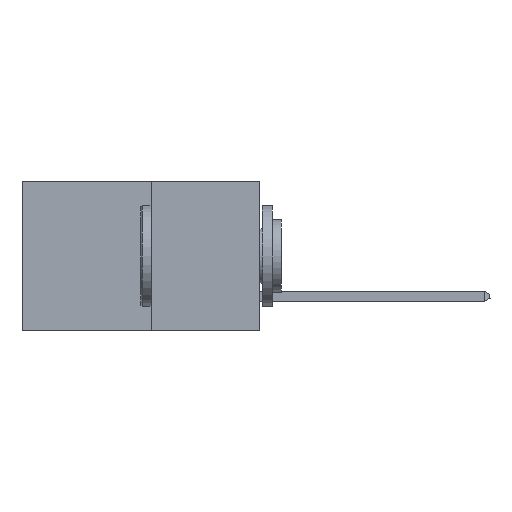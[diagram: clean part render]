
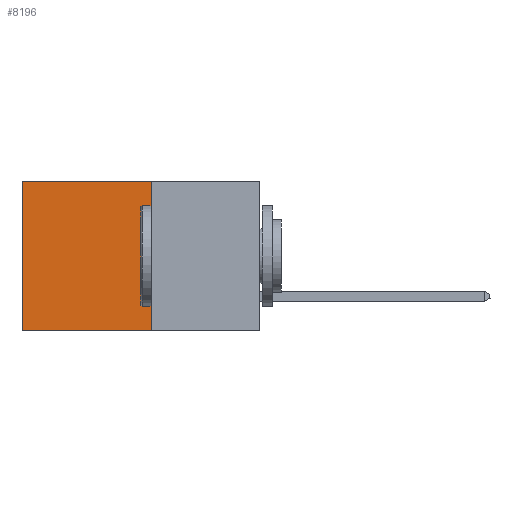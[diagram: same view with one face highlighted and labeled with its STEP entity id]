
A CAD part, left-side view. The second image highlights one B-rep face of the part: STEP entity #8196.
In plain terms, the highlighted planar face has unit normal (-1, 0, 0).
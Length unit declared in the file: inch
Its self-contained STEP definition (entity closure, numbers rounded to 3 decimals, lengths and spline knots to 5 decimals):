
#45 = CARTESIAN_POINT ( 'NONE',  ( 0.277, 0.27, 0. ) ) ;
#1614 = VECTOR ( 'NONE', #14670, 39.37008 ) ;
#1709 = CARTESIAN_POINT ( 'NONE',  ( 0.277, 0.59, 0. ) ) ;
#2320 = CARTESIAN_POINT ( 'NONE',  ( 0.277, 0.59, -0.37 ) ) ;
#2642 = EDGE_CURVE ( 'NONE', #5969, #11753, #12850, .T. ) ;
#2899 = EDGE_CURVE ( 'NONE', #5969, #7087, #11988, .T. ) ;
#3851 = EDGE_LOOP ( 'NONE', ( #8038, #6498, #10571, #11780 ) ) ;
#5511 = VERTEX_POINT ( 'NONE', #7799 ) ;
#5912 = DIRECTION ( 'NONE',  ( 0., 0., -1. ) ) ;
#5969 = VERTEX_POINT ( 'NONE', #14840 ) ;
#6498 = ORIENTED_EDGE ( 'NONE', *, *, #14004, .F. ) ;
#7087 = VERTEX_POINT ( 'NONE', #1709 ) ;
#7191 = FACE_OUTER_BOUND ( 'NONE', #3851, .T. ) ;
#7507 = CARTESIAN_POINT ( 'NONE',  ( 0.277, 0.27, -0.37 ) ) ;
#7799 = CARTESIAN_POINT ( 'NONE',  ( 0.277, 0.59, -0.37 ) ) ;
#8038 = ORIENTED_EDGE ( 'NONE', *, *, #17398, .T. ) ;
#8196 = ADVANCED_FACE ( 'NONE', ( #7191 ), #16973, .F. ) ;
#8259 = VECTOR ( 'NONE', #5912, 39.37008 ) ;
#10020 = AXIS2_PLACEMENT_3D ( 'NONE', #16842, #16813, #16790 ) ;
#10571 = ORIENTED_EDGE ( 'NONE', *, *, #2642, .F. ) ;
#11753 = VERTEX_POINT ( 'NONE', #13421 ) ;
#11780 = ORIENTED_EDGE ( 'NONE', *, *, #2899, .T. ) ;
#11988 = LINE ( 'NONE', #45, #16195 ) ;
#12850 = LINE ( 'NONE', #21275, #21290 ) ;
#13080 = LINE ( 'NONE', #2320, #8259 ) ;
#13421 = CARTESIAN_POINT ( 'NONE',  ( 0.277, 0.27, -0.37 ) ) ;
#14004 = EDGE_CURVE ( 'NONE', #11753, #5511, #16018, .T. ) ;
#14670 = DIRECTION ( 'NONE',  ( 0., 1., 0. ) ) ;
#14840 = CARTESIAN_POINT ( 'NONE',  ( 0.277, 0.27, 0. ) ) ;
#16018 = LINE ( 'NONE', #7507, #1614 ) ;
#16195 = VECTOR ( 'NONE', #19424, 39.37008 ) ;
#16790 = DIRECTION ( 'NONE',  ( 0., 0., -1. ) ) ;
#16813 = DIRECTION ( 'NONE',  ( 1., 0., 0. ) ) ;
#16842 = CARTESIAN_POINT ( 'NONE',  ( 0.277, 0.27, -0.37 ) ) ;
#16973 = PLANE ( 'NONE',  #10020 ) ;
#17398 = EDGE_CURVE ( 'NONE', #7087, #5511, #13080, .T. ) ;
#19424 = DIRECTION ( 'NONE',  ( 0., 1., 0. ) ) ;
#21275 = CARTESIAN_POINT ( 'NONE',  ( 0.277, 0.27, -0.37 ) ) ;
#21290 = VECTOR ( 'NONE', #21518, 39.37008 ) ;
#21518 = DIRECTION ( 'NONE',  ( 0., 0., -1. ) ) ;
